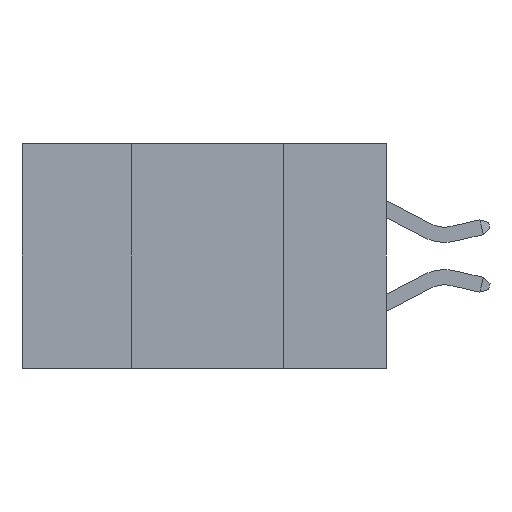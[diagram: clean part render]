
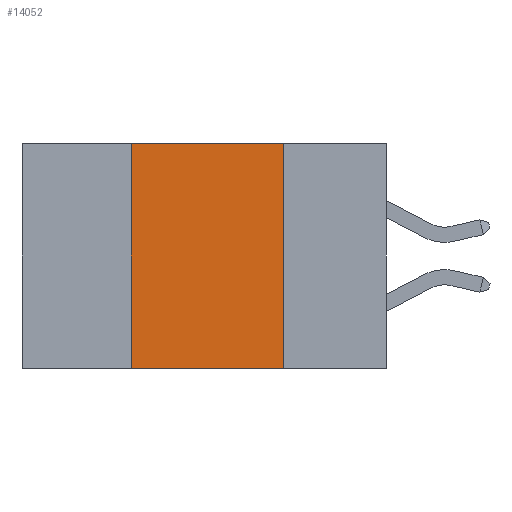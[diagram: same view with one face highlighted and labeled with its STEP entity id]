
A CAD part, left-side view. The second image highlights one B-rep face of the part: STEP entity #14052.
In plain terms, the highlighted planar face has unit normal (-1, 0, 0).
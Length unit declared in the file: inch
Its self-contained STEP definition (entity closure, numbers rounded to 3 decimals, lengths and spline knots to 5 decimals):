
#1157 = CARTESIAN_POINT ( 'NONE',  ( 0., 0.42, -0.37 ) ) ;
#1160 = PLANE ( 'NONE',  #5106 ) ;
#1641 = LINE ( 'NONE', #3054, #8067 ) ;
#1809 = CARTESIAN_POINT ( 'NONE',  ( 0., 0.17, 0. ) ) ;
#2854 = CARTESIAN_POINT ( 'NONE',  ( 0., 0.42, -0.37 ) ) ;
#2949 = DIRECTION ( 'NONE',  ( 0., 0., 1. ) ) ;
#3054 = CARTESIAN_POINT ( 'NONE',  ( 0., 0.6, -0.37 ) ) ;
#3146 = DIRECTION ( 'NONE',  ( 0., -1., 0. ) ) ;
#3772 = LINE ( 'NONE', #10581, #6790 ) ;
#3786 = DIRECTION ( 'NONE',  ( 1., 0., 0. ) ) ;
#4090 = EDGE_CURVE ( 'NONE', #12615, #6544, #3772, .T. ) ;
#4112 = ORIENTED_EDGE ( 'NONE', *, *, #4090, .F. ) ;
#4788 = EDGE_LOOP ( 'NONE', ( #4112, #13651, #10060, #6724 ) ) ;
#4867 = LINE ( 'NONE', #15909, #14340 ) ;
#5106 = AXIS2_PLACEMENT_3D ( 'NONE', #11369, #3786, #12579 ) ;
#5214 = FACE_OUTER_BOUND ( 'NONE', #4788, .T. ) ;
#5333 = LINE ( 'NONE', #2854, #14746 ) ;
#5801 = EDGE_CURVE ( 'NONE', #15914, #9160, #5333, .T. ) ;
#6285 = CARTESIAN_POINT ( 'NONE',  ( 0., 0.42, 0. ) ) ;
#6544 = VERTEX_POINT ( 'NONE', #7233 ) ;
#6724 = ORIENTED_EDGE ( 'NONE', *, *, #10563, .T. ) ;
#6773 = DIRECTION ( 'NONE',  ( 0., 0., -1. ) ) ;
#6790 = VECTOR ( 'NONE', #6773, 39.37008 ) ;
#7233 = CARTESIAN_POINT ( 'NONE',  ( 0., 0.17, -0.37 ) ) ;
#8067 = VECTOR ( 'NONE', #3146, 39.37008 ) ;
#9160 = VERTEX_POINT ( 'NONE', #6285 ) ;
#10060 = ORIENTED_EDGE ( 'NONE', *, *, #5801, .F. ) ;
#10563 = EDGE_CURVE ( 'NONE', #15914, #6544, #1641, .T. ) ;
#10581 = CARTESIAN_POINT ( 'NONE',  ( 0., 0.17, -0.37 ) ) ;
#11369 = CARTESIAN_POINT ( 'NONE',  ( 0., 0.6, 0. ) ) ;
#11723 = EDGE_CURVE ( 'NONE', #9160, #12615, #4867, .T. ) ;
#11845 = DIRECTION ( 'NONE',  ( 0., -1., 0. ) ) ;
#12579 = DIRECTION ( 'NONE',  ( 0., 0., -1. ) ) ;
#12615 = VERTEX_POINT ( 'NONE', #1809 ) ;
#13651 = ORIENTED_EDGE ( 'NONE', *, *, #11723, .F. ) ;
#14052 = ADVANCED_FACE ( 'NONE', ( #5214 ), #1160, .F. ) ;
#14340 = VECTOR ( 'NONE', #11845, 39.37008 ) ;
#14746 = VECTOR ( 'NONE', #2949, 39.37008 ) ;
#15909 = CARTESIAN_POINT ( 'NONE',  ( 0., 0.6, 0. ) ) ;
#15914 = VERTEX_POINT ( 'NONE', #1157 ) ;
